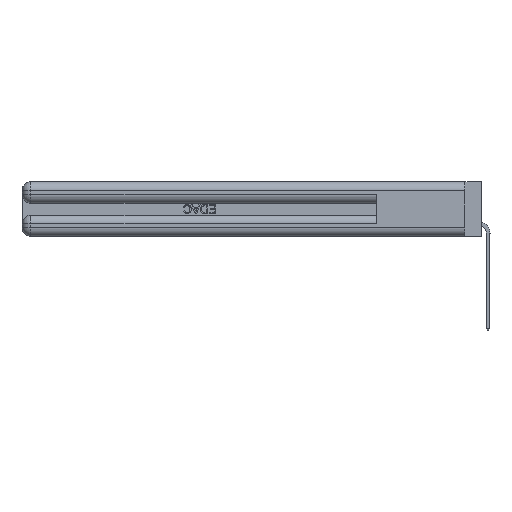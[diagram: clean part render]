
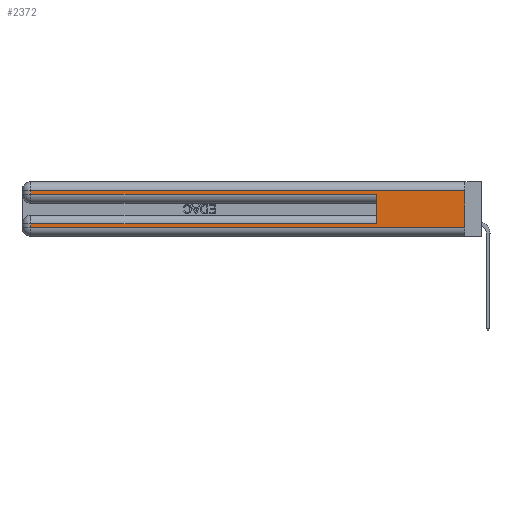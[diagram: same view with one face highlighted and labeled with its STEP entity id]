
A CAD part, left-side view. The second image highlights one B-rep face of the part: STEP entity #2372.
In plain terms, the highlighted planar face has unit normal (-1, 0, 0).
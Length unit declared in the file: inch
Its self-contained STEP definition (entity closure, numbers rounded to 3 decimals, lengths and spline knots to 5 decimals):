
#288 = EDGE_CURVE ( 'NONE', #39570, #40423, #18307, .T. ) ;
#392 = LINE ( 'NONE', #42403, #3968 ) ;
#489 = ORIENTED_EDGE ( 'NONE', *, *, #17280, .T. ) ;
#1695 = CARTESIAN_POINT ( 'NONE',  ( 0., 0.6, 0.145 ) ) ;
#2108 = FACE_OUTER_BOUND ( 'NONE', #45240, .T. ) ;
#2372 = ADVANCED_FACE ( 'NONE', ( #2108 ), #10197, .F. ) ;
#2705 = ORIENTED_EDGE ( 'NONE', *, *, #21827, .F. ) ;
#3968 = VECTOR ( 'NONE', #34998, 39.37008 ) ;
#4016 = CARTESIAN_POINT ( 'NONE',  ( 0., 2.94, 0.37 ) ) ;
#4784 = ORIENTED_EDGE ( 'NONE', *, *, #21376, .T. ) ;
#5066 = VECTOR ( 'NONE', #33305, 39.37008 ) ;
#7741 = EDGE_CURVE ( 'NONE', #22088, #45117, #12519, .T. ) ;
#8440 = VECTOR ( 'NONE', #9436, 39.37008 ) ;
#9436 = DIRECTION ( 'NONE',  ( 0., 1., 0. ) ) ;
#10197 = PLANE ( 'NONE',  #29669 ) ;
#11156 = VERTEX_POINT ( 'NONE', #44716 ) ;
#12015 = CARTESIAN_POINT ( 'NONE',  ( 0., 0., 0.085 ) ) ;
#12262 = LINE ( 'NONE', #38723, #26987 ) ;
#12519 = LINE ( 'NONE', #1695, #46118 ) ;
#12524 = LINE ( 'NONE', #12015, #8440 ) ;
#13033 = VECTOR ( 'NONE', #46287, 39.37008 ) ;
#13218 = ORIENTED_EDGE ( 'NONE', *, *, #288, .T. ) ;
#17280 = EDGE_CURVE ( 'NONE', #40423, #20682, #392, .T. ) ;
#18307 = LINE ( 'NONE', #29480, #19421 ) ;
#19421 = VECTOR ( 'NONE', #46508, 39.37008 ) ;
#19824 = LINE ( 'NONE', #28224, #37534 ) ;
#20189 = ORIENTED_EDGE ( 'NONE', *, *, #25033, .T. ) ;
#20475 = EDGE_CURVE ( 'NONE', #20936, #11156, #12262, .T. ) ;
#20609 = ORIENTED_EDGE ( 'NONE', *, *, #20475, .T. ) ;
#20682 = VERTEX_POINT ( 'NONE', #32336 ) ;
#20936 = VERTEX_POINT ( 'NONE', #35457 ) ;
#21376 = EDGE_CURVE ( 'NONE', #42317, #45117, #19824, .T. ) ;
#21827 = EDGE_CURVE ( 'NONE', #20936, #20682, #45141, .T. ) ;
#22088 = VERTEX_POINT ( 'NONE', #41864 ) ;
#23090 = DIRECTION ( 'NONE',  ( 0., 1., 0. ) ) ;
#25033 = EDGE_CURVE ( 'NONE', #11156, #42317, #37246, .T. ) ;
#26118 = ORIENTED_EDGE ( 'NONE', *, *, #7741, .F. ) ;
#26987 = VECTOR ( 'NONE', #23090, 39.37008 ) ;
#28224 = CARTESIAN_POINT ( 'NONE',  ( 0., 0., 0.285 ) ) ;
#29480 = CARTESIAN_POINT ( 'NONE',  ( 0., 2.94, 0.37 ) ) ;
#29669 = AXIS2_PLACEMENT_3D ( 'NONE', #37791, #48693, #29764 ) ;
#29764 = DIRECTION ( 'NONE',  ( 0., 0., -1. ) ) ;
#31108 = CARTESIAN_POINT ( 'NONE',  ( 0., 0.6, 0.285 ) ) ;
#31872 = ORIENTED_EDGE ( 'NONE', *, *, #32666, .T. ) ;
#32336 = CARTESIAN_POINT ( 'NONE',  ( 0., 0., 0.06 ) ) ;
#32436 = CARTESIAN_POINT ( 'NONE',  ( 0., 2.94, 0.285 ) ) ;
#32666 = EDGE_CURVE ( 'NONE', #22088, #39570, #12524, .T. ) ;
#33305 = DIRECTION ( 'NONE',  ( 0., 0., -1. ) ) ;
#33672 = CARTESIAN_POINT ( 'NONE',  ( 0., 2.94, 0.06 ) ) ;
#33918 = CARTESIAN_POINT ( 'NONE',  ( 0., 0., 0.37 ) ) ;
#34998 = DIRECTION ( 'NONE',  ( 0., -1., 0. ) ) ;
#35457 = CARTESIAN_POINT ( 'NONE',  ( 0., 0., 0.31 ) ) ;
#35535 = CARTESIAN_POINT ( 'NONE',  ( 0., 2.94, 0.085 ) ) ;
#37246 = LINE ( 'NONE', #4016, #13033 ) ;
#37534 = VECTOR ( 'NONE', #46345, 39.37008 ) ;
#37791 = CARTESIAN_POINT ( 'NONE',  ( 0., 0., 0.37 ) ) ;
#38723 = CARTESIAN_POINT ( 'NONE',  ( 0., 0., 0.31 ) ) ;
#39570 = VERTEX_POINT ( 'NONE', #35535 ) ;
#40423 = VERTEX_POINT ( 'NONE', #33672 ) ;
#41864 = CARTESIAN_POINT ( 'NONE',  ( 0., 0.6, 0.085 ) ) ;
#42317 = VERTEX_POINT ( 'NONE', #32436 ) ;
#42403 = CARTESIAN_POINT ( 'NONE',  ( 0., 0., 0.06 ) ) ;
#43488 = DIRECTION ( 'NONE',  ( 0., 0., 1. ) ) ;
#44716 = CARTESIAN_POINT ( 'NONE',  ( 0., 2.94, 0.31 ) ) ;
#45117 = VERTEX_POINT ( 'NONE', #31108 ) ;
#45141 = LINE ( 'NONE', #33918, #5066 ) ;
#45240 = EDGE_LOOP ( 'NONE', ( #2705, #20609, #20189, #4784, #26118, #31872, #13218, #489 ) ) ;
#46118 = VECTOR ( 'NONE', #43488, 39.37008 ) ;
#46287 = DIRECTION ( 'NONE',  ( 0., 0., -1. ) ) ;
#46345 = DIRECTION ( 'NONE',  ( 0., -1., 0. ) ) ;
#46508 = DIRECTION ( 'NONE',  ( 0., 0., -1. ) ) ;
#48693 = DIRECTION ( 'NONE',  ( 1., 0., 0. ) ) ;
